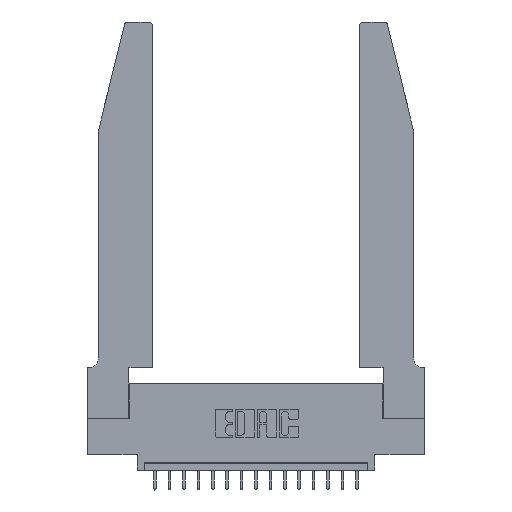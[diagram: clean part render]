
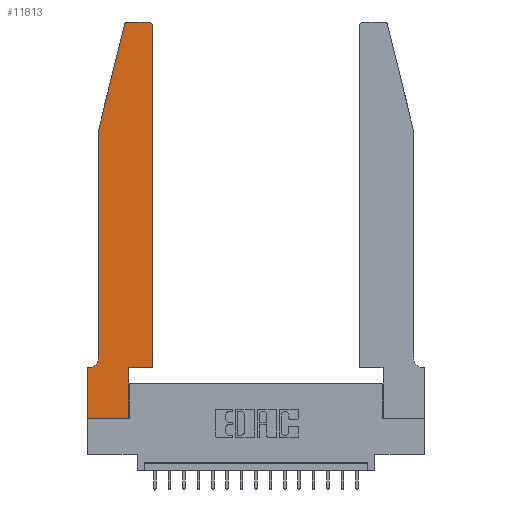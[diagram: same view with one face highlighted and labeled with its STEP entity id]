
A CAD part, top view. The second image highlights one B-rep face of the part: STEP entity #11813.
In plain terms, the highlighted planar face has unit normal (0, 0, 1).
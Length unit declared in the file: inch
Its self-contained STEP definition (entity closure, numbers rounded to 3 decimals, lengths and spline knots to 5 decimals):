
#130 = EDGE_CURVE ( 'NONE', #13081, #10834, #15862, .T. ) ;
#140 = CARTESIAN_POINT ( 'NONE',  ( 0.2605, 2.75, 0.37 ) ) ;
#537 = LINE ( 'NONE', #4698, #8572 ) ;
#550 = LINE ( 'NONE', #6298, #9654 ) ;
#1165 = VECTOR ( 'NONE', #9890, 39.37008 ) ;
#1394 = CIRCLE ( 'NONE', #9110, 0.03 ) ;
#1476 = ORIENTED_EDGE ( 'NONE', *, *, #11093, .T. ) ;
#1655 = VECTOR ( 'NONE', #2980, 39.37008 ) ;
#2086 = LINE ( 'NONE', #8126, #5900 ) ;
#2381 = AXIS2_PLACEMENT_3D ( 'NONE', #5408, #14465, #18985 ) ;
#2508 = EDGE_CURVE ( 'NONE', #11771, #19022, #9325, .T. ) ;
#2731 = DIRECTION ( 'NONE',  ( -0.239, -0.971, 0. ) ) ;
#2879 = DIRECTION ( 'NONE',  ( 1., 0., 0. ) ) ;
#2980 = DIRECTION ( 'NONE',  ( -1., 0., 0. ) ) ;
#3161 = DIRECTION ( 'NONE',  ( 1., 0., 0. ) ) ;
#3262 = DIRECTION ( 'NONE',  ( -1., 0., 0. ) ) ;
#4698 = CARTESIAN_POINT ( 'NONE',  ( 0.0755, 2., 0.37 ) ) ;
#4722 = VECTOR ( 'NONE', #3262, 39.37008 ) ;
#5141 = ORIENTED_EDGE ( 'NONE', *, *, #16870, .T. ) ;
#5205 = PLANE ( 'NONE',  #2381 ) ;
#5323 = CARTESIAN_POINT ( 'NONE',  ( 0.4505, 0.35, 0.37 ) ) ;
#5408 = CARTESIAN_POINT ( 'NONE',  ( 0., 0.35, 0.37 ) ) ;
#5499 = DIRECTION ( 'NONE',  ( 1., 0., 0. ) ) ;
#5708 = CARTESIAN_POINT ( 'NONE',  ( 0.2865, 0.35, 0.37 ) ) ;
#5762 = CARTESIAN_POINT ( 'NONE',  ( 0.0055, 0.42, 0.37 ) ) ;
#5780 = CARTESIAN_POINT ( 'NONE',  ( 0.0755, 2., 0.37 ) ) ;
#5871 = LINE ( 'NONE', #5780, #13651 ) ;
#5900 = VECTOR ( 'NONE', #14583, 39.37008 ) ;
#6298 = CARTESIAN_POINT ( 'NONE',  ( 0., 0., 0.37 ) ) ;
#6357 = CARTESIAN_POINT ( 'NONE',  ( 0., 0., 0.37 ) ) ;
#6480 = ORIENTED_EDGE ( 'NONE', *, *, #130, .T. ) ;
#6636 = AXIS2_PLACEMENT_3D ( 'NONE', #8492, #14338, #5499 ) ;
#6904 = EDGE_CURVE ( 'NONE', #9031, #9576, #550, .T. ) ;
#7207 = VERTEX_POINT ( 'NONE', #19470 ) ;
#7277 = CARTESIAN_POINT ( 'NONE',  ( 0.4505, 0.35, 0.37 ) ) ;
#7446 = DIRECTION ( 'NONE',  ( 0., 0., -1. ) ) ;
#7485 = ORIENTED_EDGE ( 'NONE', *, *, #18666, .T. ) ;
#7601 = LINE ( 'NONE', #140, #4722 ) ;
#8126 = CARTESIAN_POINT ( 'NONE',  ( 0., 0., 0.37 ) ) ;
#8203 = CIRCLE ( 'NONE', #17223, 0.07 ) ;
#8365 = VERTEX_POINT ( 'NONE', #9037 ) ;
#8456 = LINE ( 'NONE', #9862, #17111 ) ;
#8492 = CARTESIAN_POINT ( 'NONE',  ( 0.4205, 2.72, 0.37 ) ) ;
#8524 = VECTOR ( 'NONE', #15765, 39.37008 ) ;
#8572 = VECTOR ( 'NONE', #12437, 39.37008 ) ;
#8606 = CARTESIAN_POINT ( 'NONE',  ( 0.0055, 0.35, 0.37 ) ) ;
#8694 = ORIENTED_EDGE ( 'NONE', *, *, #12266, .T. ) ;
#9031 = VERTEX_POINT ( 'NONE', #6357 ) ;
#9037 = CARTESIAN_POINT ( 'NONE',  ( 0.0755, 0.42, 0.37 ) ) ;
#9066 = VERTEX_POINT ( 'NONE', #10675 ) ;
#9110 = AXIS2_PLACEMENT_3D ( 'NONE', #18587, #10826, #2879 ) ;
#9230 = EDGE_CURVE ( 'NONE', #9576, #13081, #8456, .T. ) ;
#9325 = LINE ( 'NONE', #15492, #1655 ) ;
#9427 = VERTEX_POINT ( 'NONE', #17108 ) ;
#9462 = CARTESIAN_POINT ( 'NONE',  ( 0.284, 2.75, 0.37 ) ) ;
#9576 = VERTEX_POINT ( 'NONE', #11456 ) ;
#9654 = VECTOR ( 'NONE', #3161, 39.37008 ) ;
#9812 = FACE_OUTER_BOUND ( 'NONE', #14336, .T. ) ;
#9862 = CARTESIAN_POINT ( 'NONE',  ( 0.2865, 0.35, 0.37 ) ) ;
#9890 = DIRECTION ( 'NONE',  ( 0., 1., 0. ) ) ;
#10675 = CARTESIAN_POINT ( 'NONE',  ( 0.4505, 2.72, 0.37 ) ) ;
#10758 = EDGE_CURVE ( 'NONE', #19022, #9031, #2086, .T. ) ;
#10826 = DIRECTION ( 'NONE',  ( 0., 0., 1. ) ) ;
#10834 = VERTEX_POINT ( 'NONE', #5323 ) ;
#11093 = EDGE_CURVE ( 'NONE', #12512, #9427, #1394, .T. ) ;
#11456 = CARTESIAN_POINT ( 'NONE',  ( 0.2865, 0., 0.37 ) ) ;
#11630 = ORIENTED_EDGE ( 'NONE', *, *, #2508, .T. ) ;
#11771 = VERTEX_POINT ( 'NONE', #8606 ) ;
#11776 = CIRCLE ( 'NONE', #6636, 0.03 ) ;
#11813 = ADVANCED_FACE ( 'NONE', ( #9812 ), #5205, .T. ) ;
#11912 = CARTESIAN_POINT ( 'NONE',  ( 0.4205, 2.75, 0.37 ) ) ;
#12266 = EDGE_CURVE ( 'NONE', #9427, #7207, #5871, .T. ) ;
#12437 = DIRECTION ( 'NONE',  ( 0., -1., 0. ) ) ;
#12512 = VERTEX_POINT ( 'NONE', #9462 ) ;
#13081 = VERTEX_POINT ( 'NONE', #5708 ) ;
#13371 = ORIENTED_EDGE ( 'NONE', *, *, #17109, .T. ) ;
#13651 = VECTOR ( 'NONE', #2731, 39.37008 ) ;
#14336 = EDGE_LOOP ( 'NONE', ( #18567, #1476, #8694, #5141, #16559, #11630, #16832, #16976, #18447, #6480, #13371, #7485 ) ) ;
#14338 = DIRECTION ( 'NONE',  ( 0., 0., 1. ) ) ;
#14465 = DIRECTION ( 'NONE',  ( 0., 0., 1. ) ) ;
#14506 = DIRECTION ( 'NONE',  ( 0., 1., 0. ) ) ;
#14583 = DIRECTION ( 'NONE',  ( 0., -1., 0. ) ) ;
#14715 = VERTEX_POINT ( 'NONE', #11912 ) ;
#15164 = EDGE_CURVE ( 'NONE', #8365, #11771, #8203, .T. ) ;
#15492 = CARTESIAN_POINT ( 'NONE',  ( 0.0755, 0.35, 0.37 ) ) ;
#15619 = CARTESIAN_POINT ( 'NONE',  ( 0., 0.35, 0.37 ) ) ;
#15765 = DIRECTION ( 'NONE',  ( 1., 0., 0. ) ) ;
#15862 = LINE ( 'NONE', #17265, #8524 ) ;
#16433 = DIRECTION ( 'NONE',  ( -1., 0., 0. ) ) ;
#16559 = ORIENTED_EDGE ( 'NONE', *, *, #15164, .T. ) ;
#16832 = ORIENTED_EDGE ( 'NONE', *, *, #10758, .T. ) ;
#16870 = EDGE_CURVE ( 'NONE', #7207, #8365, #537, .T. ) ;
#16976 = ORIENTED_EDGE ( 'NONE', *, *, #6904, .T. ) ;
#17108 = CARTESIAN_POINT ( 'NONE',  ( 0.25487, 2.72718, 0.37 ) ) ;
#17109 = EDGE_CURVE ( 'NONE', #10834, #9066, #19162, .T. ) ;
#17111 = VECTOR ( 'NONE', #14506, 39.37008 ) ;
#17223 = AXIS2_PLACEMENT_3D ( 'NONE', #5762, #7446, #16433 ) ;
#17265 = CARTESIAN_POINT ( 'NONE',  ( 0.4505, 0.35, 0.37 ) ) ;
#18447 = ORIENTED_EDGE ( 'NONE', *, *, #9230, .T. ) ;
#18567 = ORIENTED_EDGE ( 'NONE', *, *, #19469, .T. ) ;
#18587 = CARTESIAN_POINT ( 'NONE',  ( 0.284, 2.72, 0.37 ) ) ;
#18666 = EDGE_CURVE ( 'NONE', #9066, #14715, #11776, .T. ) ;
#18985 = DIRECTION ( 'NONE',  ( 1., 0., 0. ) ) ;
#19022 = VERTEX_POINT ( 'NONE', #15619 ) ;
#19162 = LINE ( 'NONE', #7277, #1165 ) ;
#19469 = EDGE_CURVE ( 'NONE', #14715, #12512, #7601, .T. ) ;
#19470 = CARTESIAN_POINT ( 'NONE',  ( 0.0755, 2., 0.37 ) ) ;
